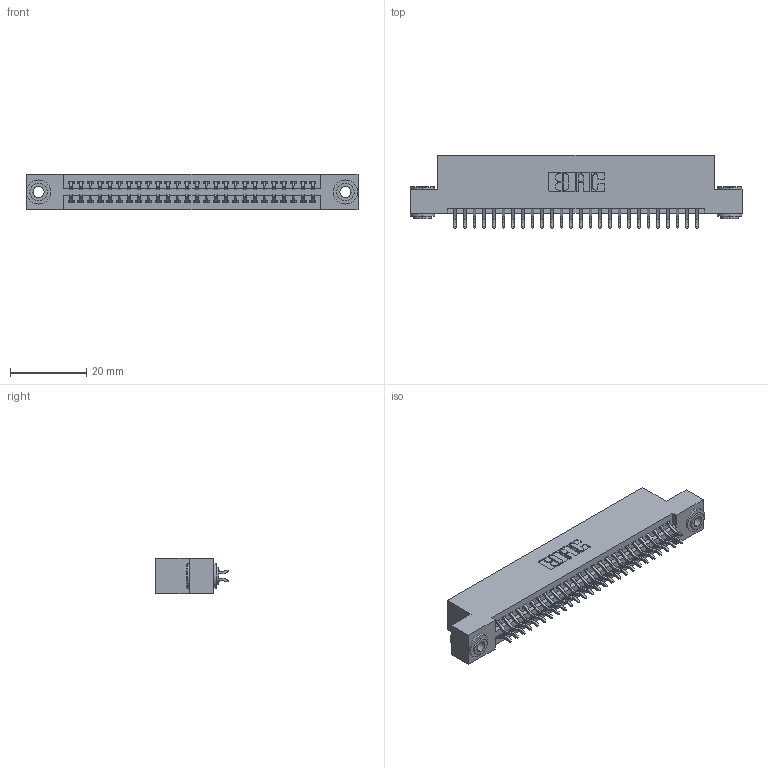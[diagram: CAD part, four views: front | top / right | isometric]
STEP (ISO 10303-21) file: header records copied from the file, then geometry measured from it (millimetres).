
FILE_DESCRIPTION (( 'STEP AP203' ), '1' );
FILE_NAME ('395-052-556-203.STEP', '2018-11-21T01:09:43', ( '' ), ( '' ), 'SwSTEP 2.0', 'SolidWorks 2016', '' );
FILE_SCHEMA (( 'CONFIG_CONTROL_DESIGN' ));
Length unit declared in the file: inch
Products named in the file (4): 345 Part_Flush Mounting Lugs - 0.156 Dia-TH; 345-250-002_345-250-002-102; 395-052-556-203; 345-292-001_556 Tail
Assembly tree (55 placements, depth 2):
  395-052-556-203
    345 Part_Flush Mounting Lugs - 0.156 Dia-TH
    345-292-001_556 Tail  x52
    345-250-002_345-250-002-102  x2
Bounding box: 87.25 x 19.24 x 9.4 mm (x, y, z)
Volume: 8344.3 mm3; surface area: 12183.7 mm2
Topology: 55 solids, 55 shells, 3076 faces, 9101 edges, 5994 vertices
Faces by surface type: plane 2014, cylinder 1054, cone 8
Entity records: 23424 total; most frequent: CARTESIAN_POINT 3931, ORIENTED_EDGE 3846, DIRECTION 3505, EDGE_CURVE 1923, VECTOR 1655, LINE 1655, VERTEX_POINT 1278, AXIS2_PLACEMENT_3D 925
